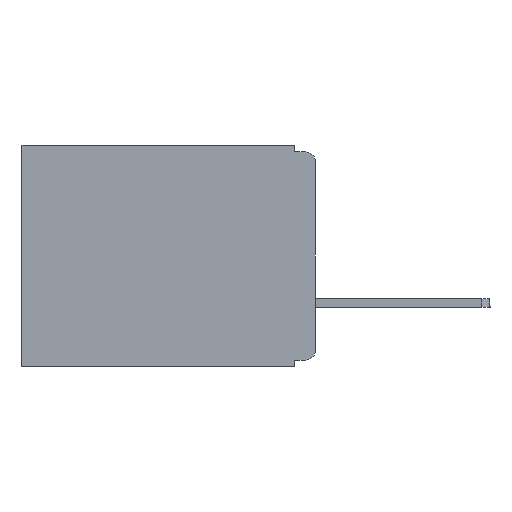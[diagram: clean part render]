
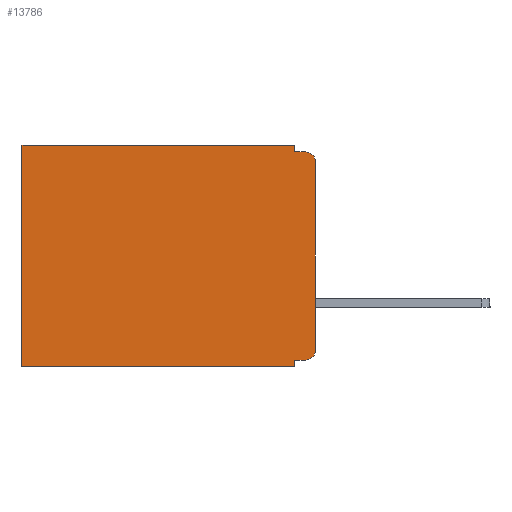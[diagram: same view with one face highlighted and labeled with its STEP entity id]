
A CAD part, left-side view. The second image highlights one B-rep face of the part: STEP entity #13786.
In plain terms, the highlighted planar face has unit normal (-1, 0, 0).
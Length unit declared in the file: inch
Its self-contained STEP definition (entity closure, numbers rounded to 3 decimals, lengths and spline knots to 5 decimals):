
#335 = ORIENTED_EDGE ( 'NONE', *, *, #11345, .F. ) ;
#379 = CARTESIAN_POINT ( 'NONE',  ( 0.3, 0.015, -0.32 ) ) ;
#1205 = LINE ( 'NONE', #9943, #17115 ) ;
#1746 = VERTEX_POINT ( 'NONE', #16874 ) ;
#1909 = DIRECTION ( 'NONE',  ( 0., 0., -1. ) ) ;
#2165 = CARTESIAN_POINT ( 'NONE',  ( 0.3, 0.031, -0.01 ) ) ;
#2216 = CIRCLE ( 'NONE', #19688, 0.015 ) ;
#2381 = LINE ( 'NONE', #5007, #18285 ) ;
#2429 = AXIS2_PLACEMENT_3D ( 'NONE', #8241, #18987, #9789 ) ;
#2476 = CARTESIAN_POINT ( 'NONE',  ( 0.3, 0., -0.01 ) ) ;
#2703 = AXIS2_PLACEMENT_3D ( 'NONE', #7477, #19778, #10575 ) ;
#2979 = VECTOR ( 'NONE', #9626, 39.37008 ) ;
#3002 = ORIENTED_EDGE ( 'NONE', *, *, #7646, .F. ) ;
#3036 = VERTEX_POINT ( 'NONE', #11492 ) ;
#3152 = LINE ( 'NONE', #2476, #19035 ) ;
#3659 = CARTESIAN_POINT ( 'NONE',  ( 0.3, 0.015, -0.305 ) ) ;
#3662 = VERTEX_POINT ( 'NONE', #13086 ) ;
#3895 = CARTESIAN_POINT ( 'NONE',  ( 0.3, 0., 0. ) ) ;
#4037 = DIRECTION ( 'NONE',  ( 0., -1., 0. ) ) ;
#4856 = LINE ( 'NONE', #12631, #12565 ) ;
#5007 = CARTESIAN_POINT ( 'NONE',  ( 0.3, 0., -0.33 ) ) ;
#5146 = FACE_OUTER_BOUND ( 'NONE', #12450, .T. ) ;
#5216 = DIRECTION ( 'NONE',  ( 0., 0., -1. ) ) ;
#5313 = ORIENTED_EDGE ( 'NONE', *, *, #15348, .T. ) ;
#5925 = PLANE ( 'NONE',  #2703 ) ;
#6055 = EDGE_CURVE ( 'NONE', #1746, #19097, #2381, .T. ) ;
#6212 = VERTEX_POINT ( 'NONE', #2165 ) ;
#6313 = CARTESIAN_POINT ( 'NONE',  ( 0.3, 0., -0.32 ) ) ;
#6533 = ORIENTED_EDGE ( 'NONE', *, *, #15280, .T. ) ;
#6590 = VECTOR ( 'NONE', #11648, 39.37008 ) ;
#6885 = VECTOR ( 'NONE', #7878, 39.37008 ) ;
#7240 = VERTEX_POINT ( 'NONE', #19103 ) ;
#7477 = CARTESIAN_POINT ( 'NONE',  ( 0.3, 0., -0.33 ) ) ;
#7489 = CIRCLE ( 'NONE', #2429, 0.015 ) ;
#7646 = EDGE_CURVE ( 'NONE', #3036, #6212, #19160, .T. ) ;
#7720 = ORIENTED_EDGE ( 'NONE', *, *, #6055, .F. ) ;
#7735 = ORIENTED_EDGE ( 'NONE', *, *, #9156, .T. ) ;
#7878 = DIRECTION ( 'NONE',  ( 0., 0., -1. ) ) ;
#8241 = CARTESIAN_POINT ( 'NONE',  ( 0.3, 0.015, -0.025 ) ) ;
#8250 = ORIENTED_EDGE ( 'NONE', *, *, #10530, .T. ) ;
#8429 = CARTESIAN_POINT ( 'NONE',  ( 0.3, 0.015, -0.01 ) ) ;
#9156 = EDGE_CURVE ( 'NONE', #3036, #7240, #14814, .T. ) ;
#9312 = LINE ( 'NONE', #6313, #17951 ) ;
#9477 = CARTESIAN_POINT ( 'NONE',  ( 0.3, 0., -0.305 ) ) ;
#9626 = DIRECTION ( 'NONE',  ( 0., 1., 0. ) ) ;
#9789 = DIRECTION ( 'NONE',  ( 0., 0., -1. ) ) ;
#9863 = EDGE_CURVE ( 'NONE', #10490, #16186, #14818, .T. ) ;
#9943 = CARTESIAN_POINT ( 'NONE',  ( 0.3, 0.031, -0.33 ) ) ;
#10220 = CARTESIAN_POINT ( 'NONE',  ( 0.3, 0.437, -0.33 ) ) ;
#10490 = VERTEX_POINT ( 'NONE', #14418 ) ;
#10530 = EDGE_CURVE ( 'NONE', #19133, #19097, #2216, .T. ) ;
#10575 = DIRECTION ( 'NONE',  ( 0., 0., -1. ) ) ;
#11345 = EDGE_CURVE ( 'NONE', #6212, #13541, #3152, .T. ) ;
#11492 = CARTESIAN_POINT ( 'NONE',  ( 0.3, 0.031, 0. ) ) ;
#11648 = DIRECTION ( 'NONE',  ( 0., 1., 0. ) ) ;
#11849 = EDGE_CURVE ( 'NONE', #3662, #10490, #1205, .T. ) ;
#12285 = DIRECTION ( 'NONE',  ( 0., 0., -1. ) ) ;
#12450 = EDGE_LOOP ( 'NONE', ( #7720, #5313, #335, #3002, #7735, #6533, #15544, #12890, #17382, #8250 ) ) ;
#12565 = VECTOR ( 'NONE', #1909, 39.37008 ) ;
#12631 = CARTESIAN_POINT ( 'NONE',  ( 0.3, 0.437, -0.33 ) ) ;
#12890 = ORIENTED_EDGE ( 'NONE', *, *, #11849, .F. ) ;
#13086 = CARTESIAN_POINT ( 'NONE',  ( 0.3, 0.031, -0.32 ) ) ;
#13541 = VERTEX_POINT ( 'NONE', #8429 ) ;
#13786 = ADVANCED_FACE ( 'NONE', ( #5146 ), #5925, .F. ) ;
#14418 = CARTESIAN_POINT ( 'NONE',  ( 0.3, 0.031, -0.33 ) ) ;
#14484 = DIRECTION ( 'NONE',  ( -1., 0., 0. ) ) ;
#14814 = LINE ( 'NONE', #3895, #6590 ) ;
#14818 = LINE ( 'NONE', #18826, #2979 ) ;
#15280 = EDGE_CURVE ( 'NONE', #7240, #16186, #4856, .T. ) ;
#15348 = EDGE_CURVE ( 'NONE', #1746, #13541, #7489, .T. ) ;
#15544 = ORIENTED_EDGE ( 'NONE', *, *, #9863, .F. ) ;
#15577 = CARTESIAN_POINT ( 'NONE',  ( 0.3, 0.031, 0. ) ) ;
#16186 = VERTEX_POINT ( 'NONE', #10220 ) ;
#16874 = CARTESIAN_POINT ( 'NONE',  ( 0.3, 0., -0.025 ) ) ;
#17085 = DIRECTION ( 'NONE',  ( 0., 1., 0. ) ) ;
#17115 = VECTOR ( 'NONE', #19213, 39.37008 ) ;
#17382 = ORIENTED_EDGE ( 'NONE', *, *, #19033, .F. ) ;
#17951 = VECTOR ( 'NONE', #17085, 39.37008 ) ;
#18285 = VECTOR ( 'NONE', #12285, 39.37008 ) ;
#18826 = CARTESIAN_POINT ( 'NONE',  ( 0.3, 0., -0.33 ) ) ;
#18987 = DIRECTION ( 'NONE',  ( -1., 0., 0. ) ) ;
#19033 = EDGE_CURVE ( 'NONE', #19133, #3662, #9312, .T. ) ;
#19035 = VECTOR ( 'NONE', #4037, 39.37008 ) ;
#19097 = VERTEX_POINT ( 'NONE', #9477 ) ;
#19103 = CARTESIAN_POINT ( 'NONE',  ( 0.3, 0.437, 0. ) ) ;
#19133 = VERTEX_POINT ( 'NONE', #379 ) ;
#19160 = LINE ( 'NONE', #15577, #6885 ) ;
#19213 = DIRECTION ( 'NONE',  ( 0., 0., -1. ) ) ;
#19688 = AXIS2_PLACEMENT_3D ( 'NONE', #3659, #14484, #5216 ) ;
#19778 = DIRECTION ( 'NONE',  ( 1., 0., 0. ) ) ;
